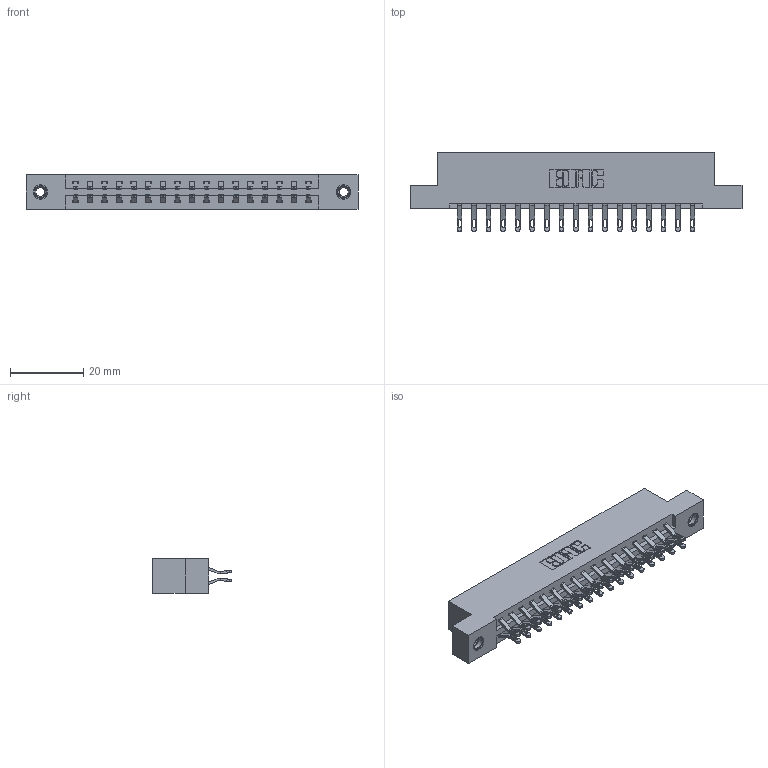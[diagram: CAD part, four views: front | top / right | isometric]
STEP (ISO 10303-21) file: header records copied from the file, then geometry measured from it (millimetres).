
FILE_DESCRIPTION (( 'STEP AP203' ), '1' );
FILE_NAME ('337-034-555-207.STEP', '2019-10-08T20:17:14', ( '' ), ( '' ), 'SwSTEP 2.0', 'SolidWorks 2016', '' );
FILE_SCHEMA (( 'CONFIG_CONTROL_DESIGN' ));
Length unit declared in the file: inch
Products named in the file (4): 345-250-001_345-250-005-103; 337 Part_Flush Mounting Lugs - 0.156 Dia-TI; 345-292-001_555 Tail; 337-034-555-207
Assembly tree (37 placements, depth 2):
  337-034-555-207
    337 Part_Flush Mounting Lugs - 0.156 Dia-TI
    345-292-001_555 Tail  x34
    345-250-001_345-250-005-103  x2
Bounding box: 90.37 x 21.47 x 9.4 mm (x, y, z)
Volume: 9276.6 mm3; surface area: 10651.9 mm2
Topology: 37 solids, 37 shells, 2214 faces, 6873 edges, 4574 vertices
Faces by surface type: plane 1326, cylinder 872, cone 12, torus 4
Entity records: 17926 total; most frequent: CARTESIAN_POINT 3055, ORIENTED_EDGE 2954, DIRECTION 2647, EDGE_CURVE 1477, VECTOR 1309, LINE 1309, VERTEX_POINT 980, AXIS2_PLACEMENT_3D 669
